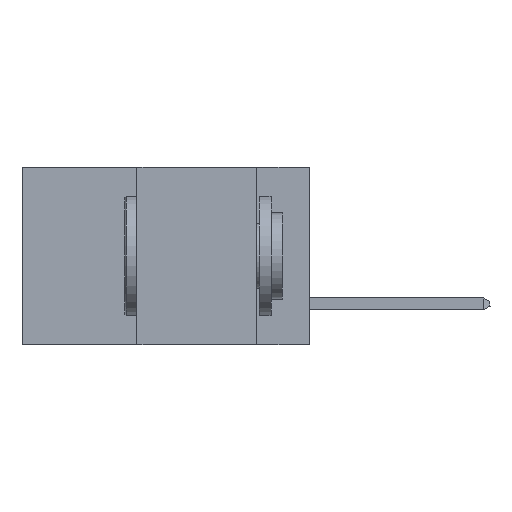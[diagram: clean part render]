
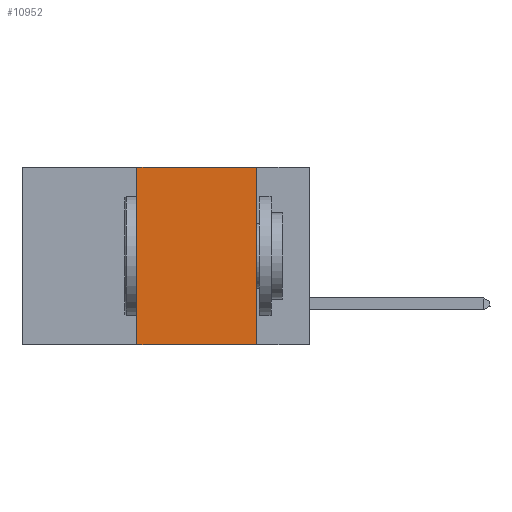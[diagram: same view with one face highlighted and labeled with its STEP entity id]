
A CAD part, left-side view. The second image highlights one B-rep face of the part: STEP entity #10952.
In plain terms, the highlighted planar face has unit normal (-1, 0, 0).
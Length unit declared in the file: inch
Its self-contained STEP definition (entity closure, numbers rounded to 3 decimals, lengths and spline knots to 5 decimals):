
#2163 = ORIENTED_EDGE ( 'NONE', *, *, #22263, .F. ) ;
#2364 = VECTOR ( 'NONE', #17062, 39.37008 ) ;
#2889 = PLANE ( 'NONE',  #7040 ) ;
#3566 = CARTESIAN_POINT ( 'NONE',  ( 0., 0.11, -0.37 ) ) ;
#5176 = EDGE_CURVE ( 'NONE', #33358, #37243, #30258, .T. ) ;
#6691 = DIRECTION ( 'NONE',  ( 0., 0., -1. ) ) ;
#7040 = AXIS2_PLACEMENT_3D ( 'NONE', #35730, #39430, #6691 ) ;
#9363 = VERTEX_POINT ( 'NONE', #16523 ) ;
#10952 = ADVANCED_FACE ( 'NONE', ( #42354 ), #2889, .F. ) ;
#11708 = CARTESIAN_POINT ( 'NONE',  ( 0., 0.11, 0. ) ) ;
#13163 = ORIENTED_EDGE ( 'NONE', *, *, #5176, .T. ) ;
#16255 = VECTOR ( 'NONE', #26545, 39.37008 ) ;
#16523 = CARTESIAN_POINT ( 'NONE',  ( 0., 0.11, 0. ) ) ;
#17062 = DIRECTION ( 'NONE',  ( 0., -1., 0. ) ) ;
#20255 = VECTOR ( 'NONE', #46438, 39.37008 ) ;
#21235 = EDGE_CURVE ( 'NONE', #40382, #9363, #23714, .T. ) ;
#21684 = CARTESIAN_POINT ( 'NONE',  ( 0., 0.6, 0. ) ) ;
#22263 = EDGE_CURVE ( 'NONE', #33358, #40382, #29958, .T. ) ;
#23714 = LINE ( 'NONE', #21684, #36324 ) ;
#24419 = CARTESIAN_POINT ( 'NONE',  ( 0., 0.36, -0.37 ) ) ;
#24616 = CARTESIAN_POINT ( 'NONE',  ( 0., 0.6, -0.37 ) ) ;
#26545 = DIRECTION ( 'NONE',  ( 0., 0., -1. ) ) ;
#27161 = LINE ( 'NONE', #11708, #16255 ) ;
#27862 = EDGE_CURVE ( 'NONE', #9363, #37243, #27161, .T. ) ;
#29785 = DIRECTION ( 'NONE',  ( 0., -1., 0. ) ) ;
#29958 = LINE ( 'NONE', #32309, #20255 ) ;
#30258 = LINE ( 'NONE', #24616, #2364 ) ;
#31004 = ORIENTED_EDGE ( 'NONE', *, *, #27862, .F. ) ;
#32309 = CARTESIAN_POINT ( 'NONE',  ( 0., 0.36, 0. ) ) ;
#33358 = VERTEX_POINT ( 'NONE', #24419 ) ;
#35730 = CARTESIAN_POINT ( 'NONE',  ( 0., 0.6, 0. ) ) ;
#36324 = VECTOR ( 'NONE', #29785, 39.37008 ) ;
#36363 = EDGE_LOOP ( 'NONE', ( #31004, #45959, #2163, #13163 ) ) ;
#37243 = VERTEX_POINT ( 'NONE', #3566 ) ;
#39430 = DIRECTION ( 'NONE',  ( 1., 0., 0. ) ) ;
#40382 = VERTEX_POINT ( 'NONE', #44262 ) ;
#42354 = FACE_OUTER_BOUND ( 'NONE', #36363, .T. ) ;
#44262 = CARTESIAN_POINT ( 'NONE',  ( 0., 0.36, 0. ) ) ;
#45959 = ORIENTED_EDGE ( 'NONE', *, *, #21235, .F. ) ;
#46438 = DIRECTION ( 'NONE',  ( 0., 0., 1. ) ) ;
